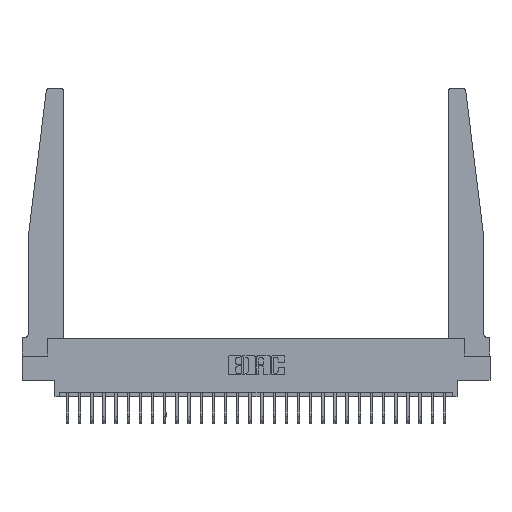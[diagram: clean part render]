
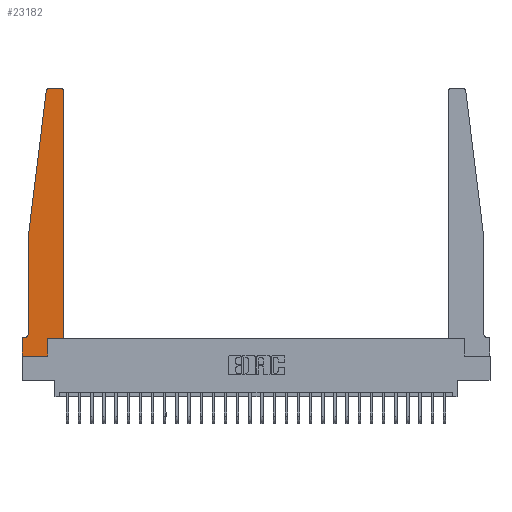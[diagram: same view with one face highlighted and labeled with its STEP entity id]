
A CAD part, top view. The second image highlights one B-rep face of the part: STEP entity #23182.
In plain terms, the highlighted planar face has unit normal (0, 0, 1).
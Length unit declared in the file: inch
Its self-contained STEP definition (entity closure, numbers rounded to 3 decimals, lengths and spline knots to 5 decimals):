
#215 = VECTOR ( 'NONE', #7315, 39.37008 ) ;
#437 = CARTESIAN_POINT ( 'NONE',  ( 0.25, 2.75, 0.37 ) ) ;
#605 = VECTOR ( 'NONE', #9693, 39.37008 ) ;
#985 = CIRCLE ( 'NONE', #14348, 0.05 ) ;
#1038 = DIRECTION ( 'NONE',  ( 1., 0., 0. ) ) ;
#1180 = CARTESIAN_POINT ( 'NONE',  ( 0., 0., 0.37 ) ) ;
#1447 = LINE ( 'NONE', #23241, #23567 ) ;
#1626 = DIRECTION ( 'NONE',  ( 1., 0., 0. ) ) ;
#2007 = CARTESIAN_POINT ( 'NONE',  ( 0.395, 2.75, 0.37 ) ) ;
#2583 = DIRECTION ( 'NONE',  ( 0., 1., 0. ) ) ;
#2769 = ORIENTED_EDGE ( 'NONE', *, *, #8329, .T. ) ;
#2799 = CARTESIAN_POINT ( 'NONE',  ( 0.065, 0.2375, 0.37 ) ) ;
#2998 = AXIS2_PLACEMENT_3D ( 'NONE', #3888, #18000, #5937 ) ;
#3274 = ORIENTED_EDGE ( 'NONE', *, *, #10268, .T. ) ;
#3291 = CARTESIAN_POINT ( 'NONE',  ( 0.065, 0.1875, 0.37 ) ) ;
#3888 = CARTESIAN_POINT ( 'NONE',  ( 0.395, 2.72, 0.37 ) ) ;
#3973 = CARTESIAN_POINT ( 'NONE',  ( 0., 0.1875, 0.37 ) ) ;
#4555 = VERTEX_POINT ( 'NONE', #19357 ) ;
#4836 = VERTEX_POINT ( 'NONE', #2007 ) ;
#5213 = ORIENTED_EDGE ( 'NONE', *, *, #12097, .T. ) ;
#5404 = CARTESIAN_POINT ( 'NONE',  ( 0.2605, 0., 0.37 ) ) ;
#5698 = VECTOR ( 'NONE', #1038, 39.37008 ) ;
#5937 = DIRECTION ( 'NONE',  ( 1., 0., 0. ) ) ;
#6761 = CARTESIAN_POINT ( 'NONE',  ( 0.015, 0.1875, 0.37 ) ) ;
#6837 = EDGE_CURVE ( 'NONE', #4836, #25720, #14384, .T. ) ;
#7233 = VERTEX_POINT ( 'NONE', #20422 ) ;
#7315 = DIRECTION ( 'NONE',  ( 1., 0., 0. ) ) ;
#7390 = EDGE_CURVE ( 'NONE', #8069, #11878, #985, .T. ) ;
#8069 = VERTEX_POINT ( 'NONE', #2799 ) ;
#8140 = DIRECTION ( 'NONE',  ( 0., 0., 1. ) ) ;
#8329 = EDGE_CURVE ( 'NONE', #25720, #14430, #11144, .T. ) ;
#8664 = EDGE_CURVE ( 'NONE', #16279, #24099, #24297, .T. ) ;
#8895 = DIRECTION ( 'NONE',  ( 0., 0., -1. ) ) ;
#9053 = EDGE_CURVE ( 'NONE', #19508, #8069, #16797, .T. ) ;
#9469 = ORIENTED_EDGE ( 'NONE', *, *, #22256, .T. ) ;
#9693 = DIRECTION ( 'NONE',  ( 0., -1., 0. ) ) ;
#10112 = AXIS2_PLACEMENT_3D ( 'NONE', #25780, #13798, #1626 ) ;
#10164 = VECTOR ( 'NONE', #2583, 39.37008 ) ;
#10268 = EDGE_CURVE ( 'NONE', #15049, #4836, #20485, .T. ) ;
#10317 = AXIS2_PLACEMENT_3D ( 'NONE', #3973, #8140, #22200 ) ;
#10379 = EDGE_CURVE ( 'NONE', #14430, #19508, #18616, .T. ) ;
#10971 = VECTOR ( 'NONE', #15368, 39.37008 ) ;
#11081 = LINE ( 'NONE', #23222, #5698 ) ;
#11144 = CIRCLE ( 'NONE', #10112, 0.03 ) ;
#11271 = ORIENTED_EDGE ( 'NONE', *, *, #6837, .T. ) ;
#11285 = CARTESIAN_POINT ( 'NONE',  ( 0.425, 0.18, 0.37 ) ) ;
#11878 = VERTEX_POINT ( 'NONE', #6761 ) ;
#12007 = VECTOR ( 'NONE', #24472, 39.37008 ) ;
#12097 = EDGE_CURVE ( 'NONE', #7233, #4555, #16306, .T. ) ;
#12615 = CARTESIAN_POINT ( 'NONE',  ( 0.425, 2.72, 0.37 ) ) ;
#12838 = ORIENTED_EDGE ( 'NONE', *, *, #7390, .T. ) ;
#13798 = DIRECTION ( 'NONE',  ( 0., 0., 1. ) ) ;
#13936 = CARTESIAN_POINT ( 'NONE',  ( 0.27653, 2.75, 0.37 ) ) ;
#14337 = CARTESIAN_POINT ( 'NONE',  ( 0.24675, 2.72367, 0.37 ) ) ;
#14348 = AXIS2_PLACEMENT_3D ( 'NONE', #20927, #8895, #22960 ) ;
#14384 = LINE ( 'NONE', #437, #24405 ) ;
#14430 = VERTEX_POINT ( 'NONE', #14337 ) ;
#14593 = ORIENTED_EDGE ( 'NONE', *, *, #19329, .T. ) ;
#14740 = CARTESIAN_POINT ( 'NONE',  ( 0.2605, 0.18, 0.37 ) ) ;
#15049 = VERTEX_POINT ( 'NONE', #12615 ) ;
#15089 = DIRECTION ( 'NONE',  ( 0., 1., 0. ) ) ;
#15165 = VECTOR ( 'NONE', #17426, 39.37008 ) ;
#15368 = DIRECTION ( 'NONE',  ( 0., -1., 0. ) ) ;
#15489 = CARTESIAN_POINT ( 'NONE',  ( 0.2605, 0.18, 0.37 ) ) ;
#15785 = LINE ( 'NONE', #11285, #215 ) ;
#16279 = VERTEX_POINT ( 'NONE', #5404 ) ;
#16306 = LINE ( 'NONE', #1180, #10971 ) ;
#16467 = ORIENTED_EDGE ( 'NONE', *, *, #8664, .T. ) ;
#16797 = LINE ( 'NONE', #17702, #605 ) ;
#17426 = DIRECTION ( 'NONE',  ( -1., 0., 0. ) ) ;
#17702 = CARTESIAN_POINT ( 'NONE',  ( 0.065, 1.25, 0.37 ) ) ;
#18000 = DIRECTION ( 'NONE',  ( 0., 0., 1. ) ) ;
#18059 = CARTESIAN_POINT ( 'NONE',  ( 0.065, 1.25, 0.37 ) ) ;
#18616 = LINE ( 'NONE', #20443, #12007 ) ;
#18778 = DIRECTION ( 'NONE',  ( -1., 0., 0. ) ) ;
#19329 = EDGE_CURVE ( 'NONE', #26049, #15049, #1447, .T. ) ;
#19357 = CARTESIAN_POINT ( 'NONE',  ( 0., 0., 0.37 ) ) ;
#19508 = VERTEX_POINT ( 'NONE', #18059 ) ;
#20097 = PLANE ( 'NONE',  #10317 ) ;
#20422 = CARTESIAN_POINT ( 'NONE',  ( 0., 0.1875, 0.37 ) ) ;
#20443 = CARTESIAN_POINT ( 'NONE',  ( 0.065, 1.25, 0.37 ) ) ;
#20451 = FACE_OUTER_BOUND ( 'NONE', #24248, .T. ) ;
#20485 = CIRCLE ( 'NONE', #2998, 0.03 ) ;
#20927 = CARTESIAN_POINT ( 'NONE',  ( 0.015, 0.2375, 0.37 ) ) ;
#21393 = ORIENTED_EDGE ( 'NONE', *, *, #9053, .T. ) ;
#22196 = EDGE_CURVE ( 'NONE', #4555, #16279, #11081, .T. ) ;
#22200 = DIRECTION ( 'NONE',  ( 1., 0., 0. ) ) ;
#22237 = EDGE_CURVE ( 'NONE', #24099, #26049, #15785, .T. ) ;
#22256 = EDGE_CURVE ( 'NONE', #11878, #7233, #25200, .T. ) ;
#22960 = DIRECTION ( 'NONE',  ( -1., 0., 0. ) ) ;
#23182 = ADVANCED_FACE ( 'NONE', ( #20451 ), #20097, .T. ) ;
#23222 = CARTESIAN_POINT ( 'NONE',  ( 0., 0., 0.37 ) ) ;
#23241 = CARTESIAN_POINT ( 'NONE',  ( 0.425, 0.18, 0.37 ) ) ;
#23336 = ORIENTED_EDGE ( 'NONE', *, *, #22196, .T. ) ;
#23567 = VECTOR ( 'NONE', #15089, 39.37008 ) ;
#23933 = ORIENTED_EDGE ( 'NONE', *, *, #22237, .T. ) ;
#24099 = VERTEX_POINT ( 'NONE', #15489 ) ;
#24248 = EDGE_LOOP ( 'NONE', ( #11271, #2769, #25894, #21393, #12838, #9469, #5213, #23336, #16467, #23933, #14593, #3274 ) ) ;
#24297 = LINE ( 'NONE', #14740, #10164 ) ;
#24405 = VECTOR ( 'NONE', #18778, 39.37008 ) ;
#24472 = DIRECTION ( 'NONE',  ( -0.122, -0.992, 0. ) ) ;
#25124 = CARTESIAN_POINT ( 'NONE',  ( 0.425, 0.18, 0.37 ) ) ;
#25200 = LINE ( 'NONE', #3291, #15165 ) ;
#25720 = VERTEX_POINT ( 'NONE', #13936 ) ;
#25780 = CARTESIAN_POINT ( 'NONE',  ( 0.27653, 2.72, 0.37 ) ) ;
#25894 = ORIENTED_EDGE ( 'NONE', *, *, #10379, .T. ) ;
#26049 = VERTEX_POINT ( 'NONE', #25124 ) ;
